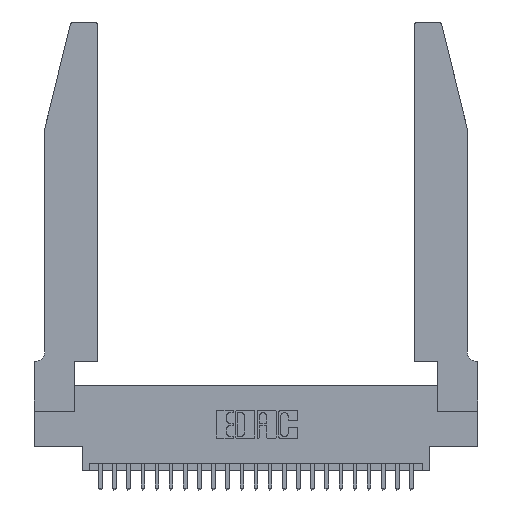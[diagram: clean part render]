
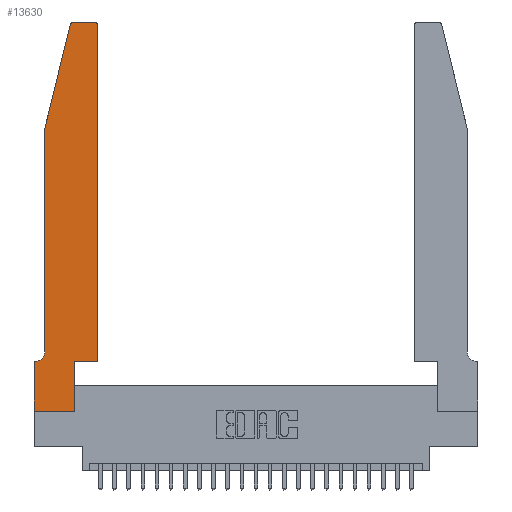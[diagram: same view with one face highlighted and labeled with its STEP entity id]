
A CAD part, top view. The second image highlights one B-rep face of the part: STEP entity #13630.
In plain terms, the highlighted planar face has unit normal (0, 0, 1).
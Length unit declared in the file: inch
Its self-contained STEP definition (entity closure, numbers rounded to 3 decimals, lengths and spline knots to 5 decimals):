
#189 = ORIENTED_EDGE ( 'NONE', *, *, #15678, .T. ) ;
#297 = PLANE ( 'NONE',  #13977 ) ;
#368 = DIRECTION ( 'NONE',  ( 1., 0., 0. ) ) ;
#394 = LINE ( 'NONE', #17071, #5121 ) ;
#584 = ORIENTED_EDGE ( 'NONE', *, *, #7315, .T. ) ;
#1065 = CARTESIAN_POINT ( 'NONE',  ( 0.0755, 2., 0.37 ) ) ;
#2230 = VERTEX_POINT ( 'NONE', #15352 ) ;
#2310 = LINE ( 'NONE', #20885, #7576 ) ;
#2313 = ORIENTED_EDGE ( 'NONE', *, *, #14583, .T. ) ;
#2515 = CARTESIAN_POINT ( 'NONE',  ( 0.284, 2.75, 0.37 ) ) ;
#3264 = DIRECTION ( 'NONE',  ( 0., -1., 0. ) ) ;
#4357 = CARTESIAN_POINT ( 'NONE',  ( 0., 0.35, 0.37 ) ) ;
#4607 = VECTOR ( 'NONE', #10777, 39.37008 ) ;
#4750 = CARTESIAN_POINT ( 'NONE',  ( 0.4205, 2.75, 0.37 ) ) ;
#4939 = DIRECTION ( 'NONE',  ( 0., -1., 0. ) ) ;
#5121 = VECTOR ( 'NONE', #3264, 39.37008 ) ;
#5298 = VERTEX_POINT ( 'NONE', #2515 ) ;
#5366 = VECTOR ( 'NONE', #4939, 39.37008 ) ;
#5563 = VERTEX_POINT ( 'NONE', #21476 ) ;
#5948 = EDGE_CURVE ( 'NONE', #15879, #19597, #24493, .T. ) ;
#6042 = ORIENTED_EDGE ( 'NONE', *, *, #14777, .T. ) ;
#6068 = LINE ( 'NONE', #1065, #21129 ) ;
#6637 = CARTESIAN_POINT ( 'NONE',  ( 0.4505, 0.35, 0.37 ) ) ;
#7155 = DIRECTION ( 'NONE',  ( -1., 0., 0. ) ) ;
#7157 = LINE ( 'NONE', #22643, #16959 ) ;
#7315 = EDGE_CURVE ( 'NONE', #2230, #15879, #15785, .T. ) ;
#7576 = VECTOR ( 'NONE', #7155, 39.37008 ) ;
#7668 = ORIENTED_EDGE ( 'NONE', *, *, #23308, .T. ) ;
#7947 = CARTESIAN_POINT ( 'NONE',  ( 0.4505, 2.72, 0.37 ) ) ;
#8072 = VERTEX_POINT ( 'NONE', #17223 ) ;
#8929 = DIRECTION ( 'NONE',  ( 0., 0., -1. ) ) ;
#8973 = VERTEX_POINT ( 'NONE', #7947 ) ;
#9169 = EDGE_CURVE ( 'NONE', #14443, #17282, #7157, .T. ) ;
#9419 = EDGE_LOOP ( 'NONE', ( #7668, #189, #24003, #584, #25219, #2313, #6042, #23271, #20513, #17723, #19270, #15908 ) ) ;
#9634 = VERTEX_POINT ( 'NONE', #4750 ) ;
#10011 = LINE ( 'NONE', #18373, #14665 ) ;
#10189 = AXIS2_PLACEMENT_3D ( 'NONE', #11132, #24843, #13133 ) ;
#10277 = CIRCLE ( 'NONE', #18884, 0.03 ) ;
#10279 = DIRECTION ( 'NONE',  ( 0., 0., 1. ) ) ;
#10290 = CARTESIAN_POINT ( 'NONE',  ( 0.2865, 0.35, 0.37 ) ) ;
#10559 = LINE ( 'NONE', #6637, #21610 ) ;
#10777 = DIRECTION ( 'NONE',  ( 1., 0., 0. ) ) ;
#11132 = CARTESIAN_POINT ( 'NONE',  ( 0.4205, 2.72, 0.37 ) ) ;
#12180 = CARTESIAN_POINT ( 'NONE',  ( 0.4505, 0.35, 0.37 ) ) ;
#12262 = DIRECTION ( 'NONE',  ( 0., 0., 1. ) ) ;
#12692 = CARTESIAN_POINT ( 'NONE',  ( 0.0755, 2., 0.37 ) ) ;
#13133 = DIRECTION ( 'NONE',  ( 1., 0., 0. ) ) ;
#13408 = VECTOR ( 'NONE', #18163, 39.37008 ) ;
#13630 = ADVANCED_FACE ( 'NONE', ( #15899 ), #297, .T. ) ;
#13977 = AXIS2_PLACEMENT_3D ( 'NONE', #4357, #10279, #24013 ) ;
#14326 = CIRCLE ( 'NONE', #10189, 0.03 ) ;
#14443 = VERTEX_POINT ( 'NONE', #22017 ) ;
#14554 = DIRECTION ( 'NONE',  ( -1., 0., 0. ) ) ;
#14583 = EDGE_CURVE ( 'NONE', #19597, #8072, #10011, .T. ) ;
#14629 = VERTEX_POINT ( 'NONE', #22532 ) ;
#14665 = VECTOR ( 'NONE', #14554, 39.37008 ) ;
#14777 = EDGE_CURVE ( 'NONE', #8072, #5563, #394, .T. ) ;
#14989 = CARTESIAN_POINT ( 'NONE',  ( 0.2865, 0., 0.37 ) ) ;
#15070 = EDGE_CURVE ( 'NONE', #19380, #14443, #23817, .T. ) ;
#15343 = EDGE_CURVE ( 'NONE', #8973, #9634, #14326, .T. ) ;
#15352 = CARTESIAN_POINT ( 'NONE',  ( 0.0755, 2., 0.37 ) ) ;
#15678 = EDGE_CURVE ( 'NONE', #5298, #14629, #10277, .T. ) ;
#15785 = LINE ( 'NONE', #12692, #5366 ) ;
#15879 = VERTEX_POINT ( 'NONE', #16685 ) ;
#15899 = FACE_OUTER_BOUND ( 'NONE', #9419, .T. ) ;
#15908 = ORIENTED_EDGE ( 'NONE', *, *, #15343, .T. ) ;
#16362 = EDGE_CURVE ( 'NONE', #17282, #8973, #10559, .T. ) ;
#16685 = CARTESIAN_POINT ( 'NONE',  ( 0.0755, 0.42, 0.37 ) ) ;
#16959 = VECTOR ( 'NONE', #24596, 39.37008 ) ;
#17071 = CARTESIAN_POINT ( 'NONE',  ( 0., 0., 0.37 ) ) ;
#17223 = CARTESIAN_POINT ( 'NONE',  ( 0., 0.35, 0.37 ) ) ;
#17282 = VERTEX_POINT ( 'NONE', #12180 ) ;
#17723 = ORIENTED_EDGE ( 'NONE', *, *, #9169, .T. ) ;
#18163 = DIRECTION ( 'NONE',  ( 0., 1., 0. ) ) ;
#18373 = CARTESIAN_POINT ( 'NONE',  ( 0.0755, 0.35, 0.37 ) ) ;
#18884 = AXIS2_PLACEMENT_3D ( 'NONE', #23989, #12262, #368 ) ;
#19270 = ORIENTED_EDGE ( 'NONE', *, *, #16362, .T. ) ;
#19380 = VERTEX_POINT ( 'NONE', #14989 ) ;
#19597 = VERTEX_POINT ( 'NONE', #22903 ) ;
#20359 = DIRECTION ( 'NONE',  ( 0., 1., 0. ) ) ;
#20513 = ORIENTED_EDGE ( 'NONE', *, *, #15070, .T. ) ;
#20701 = CARTESIAN_POINT ( 'NONE',  ( 0.0055, 0.42, 0.37 ) ) ;
#20825 = DIRECTION ( 'NONE',  ( -0.239, -0.971, 0. ) ) ;
#20885 = CARTESIAN_POINT ( 'NONE',  ( 0.2605, 2.75, 0.37 ) ) ;
#20915 = AXIS2_PLACEMENT_3D ( 'NONE', #20701, #8929, #22692 ) ;
#21129 = VECTOR ( 'NONE', #20825, 39.37008 ) ;
#21476 = CARTESIAN_POINT ( 'NONE',  ( 0., 0., 0.37 ) ) ;
#21610 = VECTOR ( 'NONE', #20359, 39.37008 ) ;
#21755 = EDGE_CURVE ( 'NONE', #5563, #19380, #24256, .T. ) ;
#22017 = CARTESIAN_POINT ( 'NONE',  ( 0.2865, 0.35, 0.37 ) ) ;
#22532 = CARTESIAN_POINT ( 'NONE',  ( 0.25487, 2.72718, 0.37 ) ) ;
#22554 = CARTESIAN_POINT ( 'NONE',  ( 0., 0., 0.37 ) ) ;
#22643 = CARTESIAN_POINT ( 'NONE',  ( 0.4505, 0.35, 0.37 ) ) ;
#22692 = DIRECTION ( 'NONE',  ( -1., 0., 0. ) ) ;
#22747 = EDGE_CURVE ( 'NONE', #14629, #2230, #6068, .T. ) ;
#22903 = CARTESIAN_POINT ( 'NONE',  ( 0.0055, 0.35, 0.37 ) ) ;
#23271 = ORIENTED_EDGE ( 'NONE', *, *, #21755, .T. ) ;
#23308 = EDGE_CURVE ( 'NONE', #9634, #5298, #2310, .T. ) ;
#23817 = LINE ( 'NONE', #10290, #13408 ) ;
#23989 = CARTESIAN_POINT ( 'NONE',  ( 0.284, 2.72, 0.37 ) ) ;
#24003 = ORIENTED_EDGE ( 'NONE', *, *, #22747, .T. ) ;
#24013 = DIRECTION ( 'NONE',  ( 1., 0., 0. ) ) ;
#24256 = LINE ( 'NONE', #22554, #4607 ) ;
#24493 = CIRCLE ( 'NONE', #20915, 0.07 ) ;
#24596 = DIRECTION ( 'NONE',  ( 1., 0., 0. ) ) ;
#24843 = DIRECTION ( 'NONE',  ( 0., 0., 1. ) ) ;
#25219 = ORIENTED_EDGE ( 'NONE', *, *, #5948, .T. ) ;
